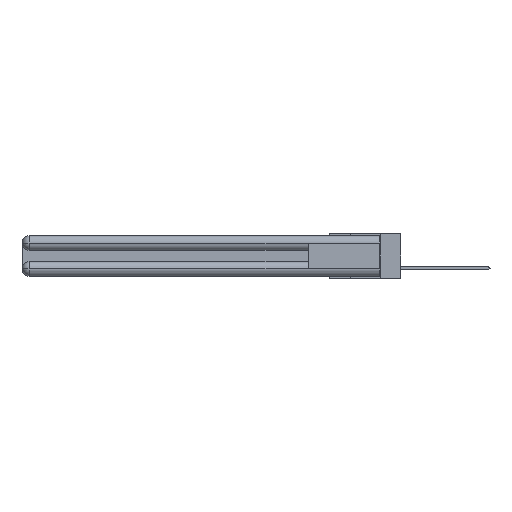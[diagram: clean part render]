
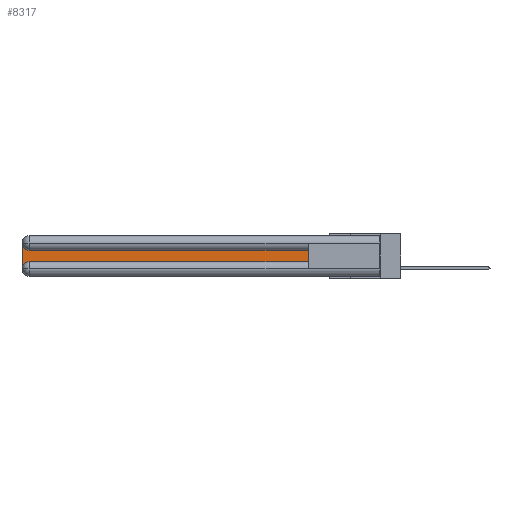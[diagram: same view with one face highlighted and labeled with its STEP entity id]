
A CAD part, left-side view. The second image highlights one B-rep face of the part: STEP entity #8317.
In plain terms, the highlighted planar face has unit normal (-1, 0, 0).
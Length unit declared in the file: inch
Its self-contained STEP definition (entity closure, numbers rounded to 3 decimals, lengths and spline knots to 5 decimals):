
#571 = EDGE_CURVE ( 'NONE', #20256, #22199, #27463, .T. ) ;
#2135 = CIRCLE ( 'NONE', #12628, 0.06 ) ;
#3974 = CARTESIAN_POINT ( 'NONE',  ( 0.075, 3., -0.1225 ) ) ;
#4013 = ORIENTED_EDGE ( 'NONE', *, *, #21907, .T. ) ;
#4246 = CARTESIAN_POINT ( 'NONE',  ( 0.075, 0.6, -0.1225 ) ) ;
#4479 = VERTEX_POINT ( 'NONE', #5849 ) ;
#4553 = CARTESIAN_POINT ( 'NONE',  ( 0.075, 3., -0.2175 ) ) ;
#5743 = CARTESIAN_POINT ( 'NONE',  ( 0.075, 2.94, -0.1225 ) ) ;
#5849 = CARTESIAN_POINT ( 'NONE',  ( 0.075, 3., -0.2775 ) ) ;
#6984 = EDGE_LOOP ( 'NONE', ( #7662, #7358, #4013, #8713, #16242, #19247 ) ) ;
#7358 = ORIENTED_EDGE ( 'NONE', *, *, #24804, .T. ) ;
#7662 = ORIENTED_EDGE ( 'NONE', *, *, #571, .T. ) ;
#8253 = CARTESIAN_POINT ( 'NONE',  ( 0.075, 0.6, -0.1225 ) ) ;
#8317 = ADVANCED_FACE ( 'NONE', ( #16354 ), #29209, .F. ) ;
#8452 = VERTEX_POINT ( 'NONE', #16085 ) ;
#8644 = DIRECTION ( 'NONE',  ( 0., 0., -1. ) ) ;
#8713 = ORIENTED_EDGE ( 'NONE', *, *, #17278, .T. ) ;
#8725 = VECTOR ( 'NONE', #24372, 39.37008 ) ;
#9155 = CARTESIAN_POINT ( 'NONE',  ( 0.075, 2.94, -0.2175 ) ) ;
#10012 = CARTESIAN_POINT ( 'NONE',  ( 0.075, 2.94, -0.2775 ) ) ;
#11065 = VERTEX_POINT ( 'NONE', #9155 ) ;
#11684 = VERTEX_POINT ( 'NONE', #12304 ) ;
#12304 = CARTESIAN_POINT ( 'NONE',  ( 0.075, 0.6, -0.2175 ) ) ;
#12628 = AXIS2_PLACEMENT_3D ( 'NONE', #24739, #17867, #8644 ) ;
#12749 = VECTOR ( 'NONE', #20528, 39.37008 ) ;
#14842 = DIRECTION ( 'NONE',  ( 0., 0., -1. ) ) ;
#15127 = EDGE_CURVE ( 'NONE', #11065, #11684, #20523, .T. ) ;
#15135 = AXIS2_PLACEMENT_3D ( 'NONE', #3974, #29313, #15482 ) ;
#15482 = DIRECTION ( 'NONE',  ( 0., 0., -1. ) ) ;
#15634 = LINE ( 'NONE', #4553, #12749 ) ;
#16085 = CARTESIAN_POINT ( 'NONE',  ( 0.075, 3., -0.0625 ) ) ;
#16242 = ORIENTED_EDGE ( 'NONE', *, *, #15127, .T. ) ;
#16354 = FACE_OUTER_BOUND ( 'NONE', #6984, .T. ) ;
#17278 = EDGE_CURVE ( 'NONE', #4479, #11065, #19133, .T. ) ;
#17687 = CARTESIAN_POINT ( 'NONE',  ( 0.075, 0.6, -0.2175 ) ) ;
#17867 = DIRECTION ( 'NONE',  ( 1., 0., 0. ) ) ;
#17939 = DIRECTION ( 'NONE',  ( 0., 1., 0. ) ) ;
#19133 = CIRCLE ( 'NONE', #23326, 0.06 ) ;
#19247 = ORIENTED_EDGE ( 'NONE', *, *, #22672, .T. ) ;
#20256 = VERTEX_POINT ( 'NONE', #8253 ) ;
#20523 = LINE ( 'NONE', #17687, #8725 ) ;
#20528 = DIRECTION ( 'NONE',  ( 0., 0., -1. ) ) ;
#20571 = LINE ( 'NONE', #24613, #22734 ) ;
#21432 = DIRECTION ( 'NONE',  ( 1., 0., 0. ) ) ;
#21907 = EDGE_CURVE ( 'NONE', #8452, #4479, #15634, .T. ) ;
#22199 = VERTEX_POINT ( 'NONE', #5743 ) ;
#22304 = DIRECTION ( 'NONE',  ( 0., 0., 1. ) ) ;
#22672 = EDGE_CURVE ( 'NONE', #11684, #20256, #20571, .T. ) ;
#22734 = VECTOR ( 'NONE', #22304, 39.37008 ) ;
#23326 = AXIS2_PLACEMENT_3D ( 'NONE', #10012, #21432, #14842 ) ;
#24372 = DIRECTION ( 'NONE',  ( 0., -1., 0. ) ) ;
#24613 = CARTESIAN_POINT ( 'NONE',  ( 0.075, 0.6, -0.2175 ) ) ;
#24739 = CARTESIAN_POINT ( 'NONE',  ( 0.075, 2.94, -0.0625 ) ) ;
#24804 = EDGE_CURVE ( 'NONE', #22199, #8452, #2135, .T. ) ;
#25687 = VECTOR ( 'NONE', #17939, 39.37008 ) ;
#27463 = LINE ( 'NONE', #4246, #25687 ) ;
#29209 = PLANE ( 'NONE',  #15135 ) ;
#29313 = DIRECTION ( 'NONE',  ( 1., 0., 0. ) ) ;
